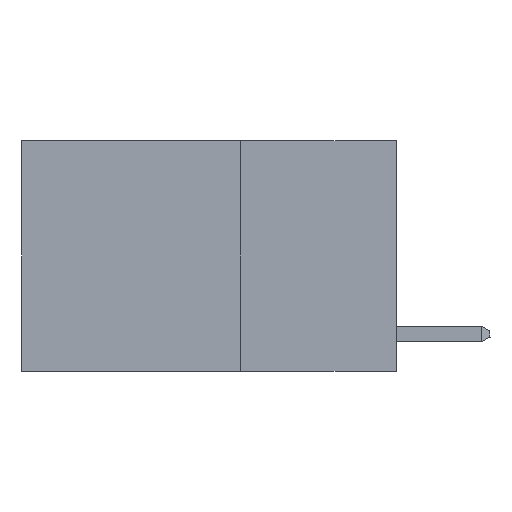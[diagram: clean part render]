
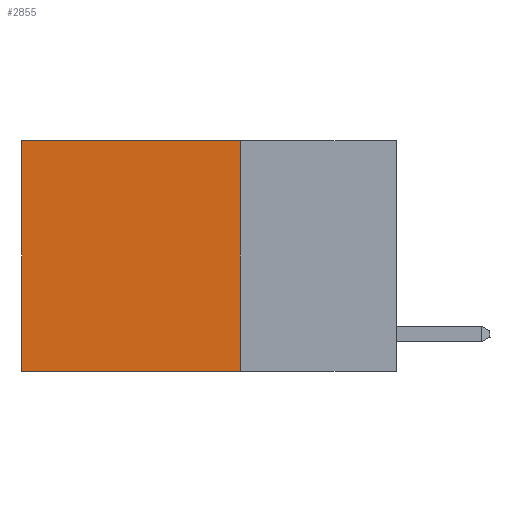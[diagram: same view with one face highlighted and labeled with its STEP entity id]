
A CAD part, left-side view. The second image highlights one B-rep face of the part: STEP entity #2855.
In plain terms, the highlighted planar face has unit normal (-1, 0, 0).
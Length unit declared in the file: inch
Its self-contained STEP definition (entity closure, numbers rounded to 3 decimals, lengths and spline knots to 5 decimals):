
#2055 = CARTESIAN_POINT ( 'NONE',  ( 0.2625, 0.6, 0. ) ) ;
#2190 = LINE ( 'NONE', #5413, #10577 ) ;
#2471 = VERTEX_POINT ( 'NONE', #18137 ) ;
#2855 = ADVANCED_FACE ( 'NONE', ( #19390 ), #17644, .F. ) ;
#2935 = VERTEX_POINT ( 'NONE', #19568 ) ;
#4090 = DIRECTION ( 'NONE',  ( 0., 1., 0. ) ) ;
#4163 = DIRECTION ( 'NONE',  ( 0., 0., -1. ) ) ;
#5413 = CARTESIAN_POINT ( 'NONE',  ( 0.2625, 0.25, 0. ) ) ;
#6694 = VERTEX_POINT ( 'NONE', #20415 ) ;
#7115 = DIRECTION ( 'NONE',  ( 0., 1., 0. ) ) ;
#7571 = DIRECTION ( 'NONE',  ( 1., 0., 0. ) ) ;
#8259 = ORIENTED_EDGE ( 'NONE', *, *, #13808, .T. ) ;
#10369 = CARTESIAN_POINT ( 'NONE',  ( 0.2625, 0.6, 0. ) ) ;
#10577 = VECTOR ( 'NONE', #7115, 39.37008 ) ;
#12460 = CARTESIAN_POINT ( 'NONE',  ( 0.2625, 0.25, -0.37 ) ) ;
#12529 = CARTESIAN_POINT ( 'NONE',  ( 0.2625, 0.25, 0. ) ) ;
#12566 = CARTESIAN_POINT ( 'NONE',  ( 0.2625, 0.25, 0. ) ) ;
#12802 = LINE ( 'NONE', #10369, #16763 ) ;
#13808 = EDGE_CURVE ( 'NONE', #16458, #6694, #12802, .T. ) ;
#13879 = ORIENTED_EDGE ( 'NONE', *, *, #19492, .F. ) ;
#14572 = EDGE_CURVE ( 'NONE', #2935, #2471, #20173, .T. ) ;
#15431 = DIRECTION ( 'NONE',  ( 0., 0., -1. ) ) ;
#16380 = VECTOR ( 'NONE', #4090, 39.37008 ) ;
#16458 = VERTEX_POINT ( 'NONE', #2055 ) ;
#16681 = EDGE_LOOP ( 'NONE', ( #8259, #13879, #18061, #21432 ) ) ;
#16763 = VECTOR ( 'NONE', #15431, 39.37008 ) ;
#17644 = PLANE ( 'NONE',  #20569 ) ;
#18061 = ORIENTED_EDGE ( 'NONE', *, *, #14572, .F. ) ;
#18137 = CARTESIAN_POINT ( 'NONE',  ( 0.2625, 0.25, -0.37 ) ) ;
#19337 = DIRECTION ( 'NONE',  ( 0., 0., -1. ) ) ;
#19346 = EDGE_CURVE ( 'NONE', #2935, #16458, #2190, .T. ) ;
#19390 = FACE_OUTER_BOUND ( 'NONE', #16681, .T. ) ;
#19492 = EDGE_CURVE ( 'NONE', #2471, #6694, #20823, .T. ) ;
#19568 = CARTESIAN_POINT ( 'NONE',  ( 0.2625, 0.25, 0. ) ) ;
#19663 = VECTOR ( 'NONE', #4163, 39.37008 ) ;
#20173 = LINE ( 'NONE', #12529, #19663 ) ;
#20415 = CARTESIAN_POINT ( 'NONE',  ( 0.2625, 0.6, -0.37 ) ) ;
#20569 = AXIS2_PLACEMENT_3D ( 'NONE', #12566, #7571, #19337 ) ;
#20823 = LINE ( 'NONE', #12460, #16380 ) ;
#21432 = ORIENTED_EDGE ( 'NONE', *, *, #19346, .T. ) ;
